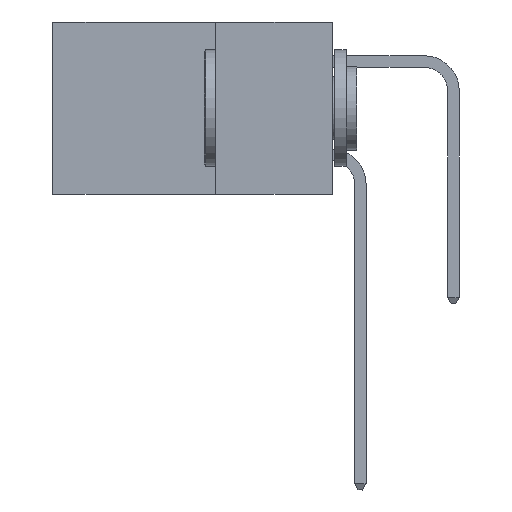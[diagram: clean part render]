
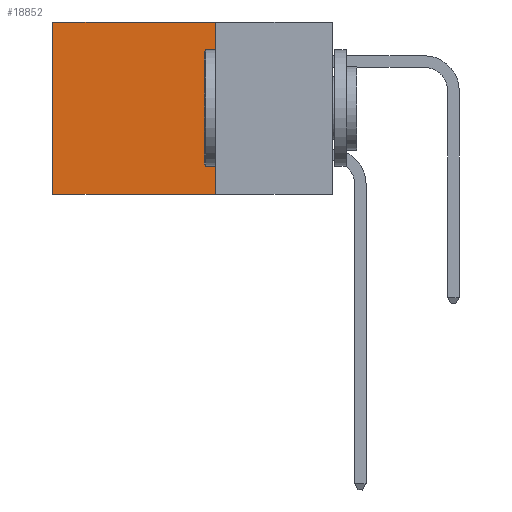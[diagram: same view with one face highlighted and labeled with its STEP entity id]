
A CAD part, left-side view. The second image highlights one B-rep face of the part: STEP entity #18852.
In plain terms, the highlighted planar face has unit normal (-1, 0, 0).
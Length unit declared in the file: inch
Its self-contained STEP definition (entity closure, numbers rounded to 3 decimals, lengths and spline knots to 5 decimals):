
#270 = ORIENTED_EDGE ( 'NONE', *, *, #6460, .F. ) ;
#1009 = LINE ( 'NONE', #11558, #17879 ) ;
#1137 = EDGE_CURVE ( 'NONE', #5163, #8903, #1009, .T. ) ;
#1204 = VERTEX_POINT ( 'NONE', #19968 ) ;
#2087 = ORIENTED_EDGE ( 'NONE', *, *, #4575, .F. ) ;
#2092 = CARTESIAN_POINT ( 'NONE',  ( 0.298, 0.25, -0.37 ) ) ;
#2300 = CARTESIAN_POINT ( 'NONE',  ( 0.298, 0.25, 0. ) ) ;
#2385 = FACE_OUTER_BOUND ( 'NONE', #11401, .T. ) ;
#2984 = CARTESIAN_POINT ( 'NONE',  ( 0.298, 0.6, 0. ) ) ;
#3601 = DIRECTION ( 'NONE',  ( 0., 1., 0. ) ) ;
#3885 = DIRECTION ( 'NONE',  ( 0., 0., -1. ) ) ;
#3957 = PLANE ( 'NONE',  #11022 ) ;
#4575 = EDGE_CURVE ( 'NONE', #5163, #15453, #10305, .T. ) ;
#5163 = VERTEX_POINT ( 'NONE', #8386 ) ;
#6460 = EDGE_CURVE ( 'NONE', #15453, #1204, #7397, .T. ) ;
#6661 = CARTESIAN_POINT ( 'NONE',  ( 0.298, 0.25, -0.37 ) ) ;
#6856 = ORIENTED_EDGE ( 'NONE', *, *, #1137, .T. ) ;
#7397 = LINE ( 'NONE', #6661, #9179 ) ;
#7448 = VECTOR ( 'NONE', #11105, 39.37008 ) ;
#8298 = DIRECTION ( 'NONE',  ( 0., 1., 0. ) ) ;
#8386 = CARTESIAN_POINT ( 'NONE',  ( 0.298, 0.25, 0. ) ) ;
#8538 = DIRECTION ( 'NONE',  ( 0., 0., -1. ) ) ;
#8679 = CARTESIAN_POINT ( 'NONE',  ( 0.298, 0.6, 0. ) ) ;
#8903 = VERTEX_POINT ( 'NONE', #8679 ) ;
#9179 = VECTOR ( 'NONE', #8298, 39.37008 ) ;
#10305 = LINE ( 'NONE', #18172, #17079 ) ;
#11022 = AXIS2_PLACEMENT_3D ( 'NONE', #2300, #18551, #3885 ) ;
#11105 = DIRECTION ( 'NONE',  ( 0., 0., -1. ) ) ;
#11401 = EDGE_LOOP ( 'NONE', ( #14509, #270, #2087, #6856 ) ) ;
#11558 = CARTESIAN_POINT ( 'NONE',  ( 0.298, 0.25, 0. ) ) ;
#12520 = LINE ( 'NONE', #2984, #7448 ) ;
#14509 = ORIENTED_EDGE ( 'NONE', *, *, #18052, .T. ) ;
#15453 = VERTEX_POINT ( 'NONE', #2092 ) ;
#17079 = VECTOR ( 'NONE', #8538, 39.37008 ) ;
#17879 = VECTOR ( 'NONE', #3601, 39.37008 ) ;
#18052 = EDGE_CURVE ( 'NONE', #8903, #1204, #12520, .T. ) ;
#18172 = CARTESIAN_POINT ( 'NONE',  ( 0.298, 0.25, 0. ) ) ;
#18551 = DIRECTION ( 'NONE',  ( 1., 0., 0. ) ) ;
#18852 = ADVANCED_FACE ( 'NONE', ( #2385 ), #3957, .F. ) ;
#19968 = CARTESIAN_POINT ( 'NONE',  ( 0.298, 0.6, -0.37 ) ) ;
